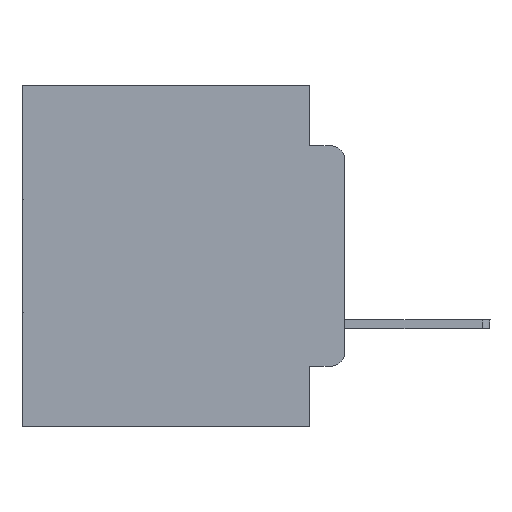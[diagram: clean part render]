
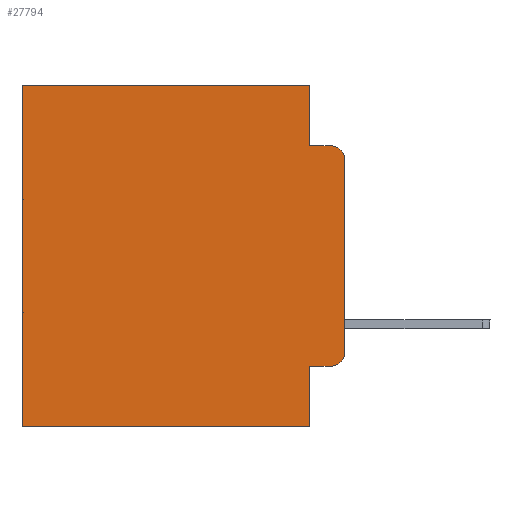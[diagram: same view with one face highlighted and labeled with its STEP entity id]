
A CAD part, left-side view. The second image highlights one B-rep face of the part: STEP entity #27794.
In plain terms, the highlighted planar face has unit normal (-1, 0, 0).
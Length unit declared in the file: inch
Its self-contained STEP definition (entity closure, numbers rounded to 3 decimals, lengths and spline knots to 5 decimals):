
#1165 = CARTESIAN_POINT ( 'NONE',  ( 0.298, 0.051, 0. ) ) ;
#1477 = DIRECTION ( 'NONE',  ( 0., 0., -1. ) ) ;
#2666 = CARTESIAN_POINT ( 'NONE',  ( 0.298, 0.473, -0.5 ) ) ;
#3177 = VECTOR ( 'NONE', #29423, 39.37008 ) ;
#3406 = VERTEX_POINT ( 'NONE', #2666 ) ;
#3630 = CARTESIAN_POINT ( 'NONE',  ( 0.298, 0., -0.5 ) ) ;
#4051 = CARTESIAN_POINT ( 'NONE',  ( 0.298, 0.051, 0. ) ) ;
#4640 = EDGE_CURVE ( 'NONE', #5524, #28916, #21359, .T. ) ;
#4854 = DIRECTION ( 'NONE',  ( -1., 0., 0. ) ) ;
#4975 = VERTEX_POINT ( 'NONE', #16594 ) ;
#5007 = CIRCLE ( 'NONE', #7909, 0.02 ) ;
#5409 = CARTESIAN_POINT ( 'NONE',  ( 0.298, 0., 0. ) ) ;
#5524 = VERTEX_POINT ( 'NONE', #1165 ) ;
#5610 = DIRECTION ( 'NONE',  ( 0., 1., 0. ) ) ;
#6198 = ORIENTED_EDGE ( 'NONE', *, *, #10833, .F. ) ;
#6231 = VECTOR ( 'NONE', #16160, 39.37008 ) ;
#6758 = VERTEX_POINT ( 'NONE', #23671 ) ;
#7909 = AXIS2_PLACEMENT_3D ( 'NONE', #16675, #12158, #24047 ) ;
#8639 = LINE ( 'NONE', #17667, #3177 ) ;
#8660 = EDGE_CURVE ( 'NONE', #17977, #25158, #15357, .T. ) ;
#9103 = CARTESIAN_POINT ( 'NONE',  ( 0.298, 0.02, -0.1085 ) ) ;
#9234 = ORIENTED_EDGE ( 'NONE', *, *, #13045, .F. ) ;
#9689 = CARTESIAN_POINT ( 'NONE',  ( 0.298, 0.051, -0.0885 ) ) ;
#10498 = CARTESIAN_POINT ( 'NONE',  ( 0.298, 0.02, -0.4115 ) ) ;
#10753 = AXIS2_PLACEMENT_3D ( 'NONE', #5409, #26342, #14742 ) ;
#10833 = EDGE_CURVE ( 'NONE', #6758, #14935, #15443, .T. ) ;
#11515 = LINE ( 'NONE', #20686, #6231 ) ;
#12086 = ORIENTED_EDGE ( 'NONE', *, *, #14259, .F. ) ;
#12158 = DIRECTION ( 'NONE',  ( -1., 0., 0. ) ) ;
#12195 = FACE_OUTER_BOUND ( 'NONE', #21540, .T. ) ;
#13045 = EDGE_CURVE ( 'NONE', #17828, #4975, #22019, .T. ) ;
#13373 = VECTOR ( 'NONE', #1477, 39.37008 ) ;
#13447 = VECTOR ( 'NONE', #5610, 39.37008 ) ;
#13602 = ORIENTED_EDGE ( 'NONE', *, *, #28135, .T. ) ;
#14083 = ORIENTED_EDGE ( 'NONE', *, *, #20464, .F. ) ;
#14259 = EDGE_CURVE ( 'NONE', #5524, #17828, #8639, .T. ) ;
#14661 = CIRCLE ( 'NONE', #23801, 0.02 ) ;
#14742 = DIRECTION ( 'NONE',  ( 0., 0., -1. ) ) ;
#14935 = VERTEX_POINT ( 'NONE', #20477 ) ;
#15357 = LINE ( 'NONE', #4051, #13373 ) ;
#15443 = LINE ( 'NONE', #19796, #28523 ) ;
#16160 = DIRECTION ( 'NONE',  ( 0., -1., 0. ) ) ;
#16594 = CARTESIAN_POINT ( 'NONE',  ( 0.298, 0.02, -0.0885 ) ) ;
#16675 = CARTESIAN_POINT ( 'NONE',  ( 0.298, 0.02, -0.3915 ) ) ;
#17026 = DIRECTION ( 'NONE',  ( 0., 0., -1. ) ) ;
#17157 = PLANE ( 'NONE',  #10753 ) ;
#17667 = CARTESIAN_POINT ( 'NONE',  ( 0.298, 0.051, 0. ) ) ;
#17828 = VERTEX_POINT ( 'NONE', #9689 ) ;
#17857 = DIRECTION ( 'NONE',  ( 0., 0., -1. ) ) ;
#17977 = VERTEX_POINT ( 'NONE', #29101 ) ;
#18266 = VERTEX_POINT ( 'NONE', #10498 ) ;
#18361 = DIRECTION ( 'NONE',  ( 0., -1., 0. ) ) ;
#18708 = ORIENTED_EDGE ( 'NONE', *, *, #8660, .F. ) ;
#19025 = LINE ( 'NONE', #3630, #13447 ) ;
#19767 = ORIENTED_EDGE ( 'NONE', *, *, #21734, .T. ) ;
#19796 = CARTESIAN_POINT ( 'NONE',  ( 0.298, 0., 0. ) ) ;
#20303 = EDGE_CURVE ( 'NONE', #17977, #18266, #11515, .T. ) ;
#20464 = EDGE_CURVE ( 'NONE', #25158, #3406, #19025, .T. ) ;
#20477 = CARTESIAN_POINT ( 'NONE',  ( 0.298, 0., -0.3915 ) ) ;
#20686 = CARTESIAN_POINT ( 'NONE',  ( 0.298, 0.051, -0.4115 ) ) ;
#21359 = LINE ( 'NONE', #23917, #25933 ) ;
#21508 = DIRECTION ( 'NONE',  ( 0., 1., 0. ) ) ;
#21540 = EDGE_LOOP ( 'NONE', ( #6198, #29124, #9234, #12086, #24983, #19767, #14083, #18708, #29552, #13602 ) ) ;
#21691 = LINE ( 'NONE', #23652, #27464 ) ;
#21734 = EDGE_CURVE ( 'NONE', #28916, #3406, #21691, .T. ) ;
#22019 = LINE ( 'NONE', #22319, #29606 ) ;
#22319 = CARTESIAN_POINT ( 'NONE',  ( 0.298, 0.051, -0.0885 ) ) ;
#22779 = CARTESIAN_POINT ( 'NONE',  ( 0.298, 0.473, 0. ) ) ;
#23652 = CARTESIAN_POINT ( 'NONE',  ( 0.298, 0.473, 0. ) ) ;
#23671 = CARTESIAN_POINT ( 'NONE',  ( 0.298, 0., -0.1085 ) ) ;
#23801 = AXIS2_PLACEMENT_3D ( 'NONE', #9103, #4854, #27470 ) ;
#23917 = CARTESIAN_POINT ( 'NONE',  ( 0.298, 0., 0. ) ) ;
#24047 = DIRECTION ( 'NONE',  ( 0., 0., -1. ) ) ;
#24983 = ORIENTED_EDGE ( 'NONE', *, *, #4640, .T. ) ;
#25158 = VERTEX_POINT ( 'NONE', #29596 ) ;
#25933 = VECTOR ( 'NONE', #21508, 39.37008 ) ;
#26342 = DIRECTION ( 'NONE',  ( 1., 0., 0. ) ) ;
#27464 = VECTOR ( 'NONE', #17026, 39.37008 ) ;
#27470 = DIRECTION ( 'NONE',  ( 0., 0., -1. ) ) ;
#27794 = ADVANCED_FACE ( 'NONE', ( #12195 ), #17157, .F. ) ;
#28135 = EDGE_CURVE ( 'NONE', #18266, #14935, #5007, .T. ) ;
#28523 = VECTOR ( 'NONE', #17857, 39.37008 ) ;
#28916 = VERTEX_POINT ( 'NONE', #22779 ) ;
#29005 = EDGE_CURVE ( 'NONE', #6758, #4975, #14661, .T. ) ;
#29101 = CARTESIAN_POINT ( 'NONE',  ( 0.298, 0.051, -0.4115 ) ) ;
#29124 = ORIENTED_EDGE ( 'NONE', *, *, #29005, .T. ) ;
#29423 = DIRECTION ( 'NONE',  ( 0., 0., -1. ) ) ;
#29552 = ORIENTED_EDGE ( 'NONE', *, *, #20303, .T. ) ;
#29596 = CARTESIAN_POINT ( 'NONE',  ( 0.298, 0.051, -0.5 ) ) ;
#29606 = VECTOR ( 'NONE', #18361, 39.37008 ) ;
